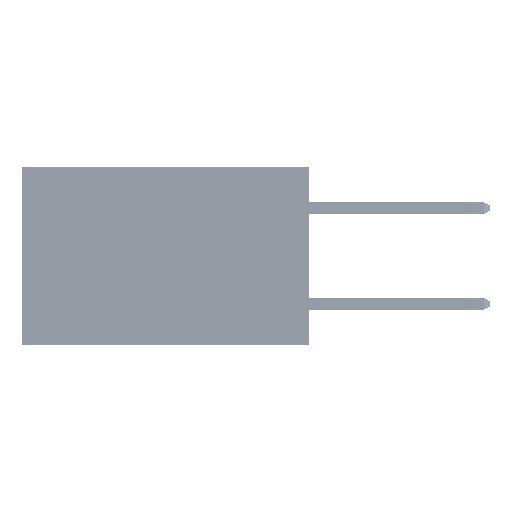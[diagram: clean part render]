
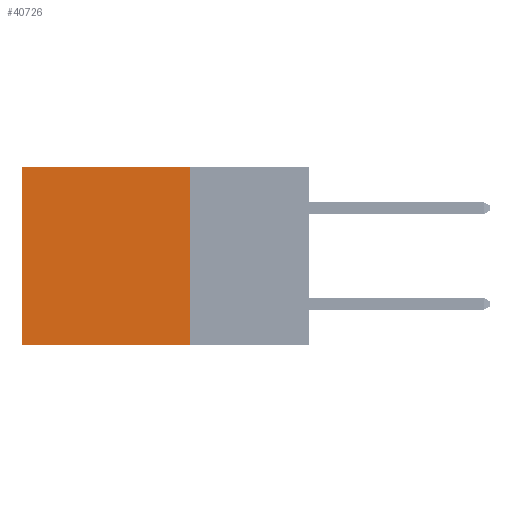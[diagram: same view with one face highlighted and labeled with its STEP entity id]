
A CAD part, left-side view. The second image highlights one B-rep face of the part: STEP entity #40726.
In plain terms, the highlighted planar face has unit normal (-1, 0, 0).
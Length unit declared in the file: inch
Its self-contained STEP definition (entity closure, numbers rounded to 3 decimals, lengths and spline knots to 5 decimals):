
#345 = ORIENTED_EDGE ( 'NONE', *, *, #44651, .F. ) ;
#456 = LINE ( 'NONE', #30104, #5459 ) ;
#1568 = CARTESIAN_POINT ( 'NONE',  ( 0.2875, 0.25, 0. ) ) ;
#2013 = LINE ( 'NONE', #16965, #23790 ) ;
#3012 = EDGE_LOOP ( 'NONE', ( #31496, #41289, #345, #5536 ) ) ;
#5459 = VECTOR ( 'NONE', #45035, 39.37008 ) ;
#5536 = ORIENTED_EDGE ( 'NONE', *, *, #22807, .T. ) ;
#8009 = VERTEX_POINT ( 'NONE', #40528 ) ;
#8767 = CARTESIAN_POINT ( 'NONE',  ( 0.2875, 0.25, -0.37 ) ) ;
#8848 = DIRECTION ( 'NONE',  ( 0., 0., -1. ) ) ;
#9375 = EDGE_CURVE ( 'NONE', #11975, #38595, #456, .T. ) ;
#11975 = VERTEX_POINT ( 'NONE', #8767 ) ;
#13280 = DIRECTION ( 'NONE',  ( 0., 0., -1. ) ) ;
#14042 = LINE ( 'NONE', #26265, #38725 ) ;
#16034 = DIRECTION ( 'NONE',  ( 0., 1., 0. ) ) ;
#16965 = CARTESIAN_POINT ( 'NONE',  ( 0.2875, 0.6, 0. ) ) ;
#17728 = DIRECTION ( 'NONE',  ( 0., 0., -1. ) ) ;
#22190 = CARTESIAN_POINT ( 'NONE',  ( 0.2875, 0.6, -0.37 ) ) ;
#22807 = EDGE_CURVE ( 'NONE', #28123, #8009, #42220, .T. ) ;
#23790 = VECTOR ( 'NONE', #13280, 39.37008 ) ;
#24289 = DIRECTION ( 'NONE',  ( 1., 0., 0. ) ) ;
#25136 = VECTOR ( 'NONE', #16034, 39.37008 ) ;
#26065 = EDGE_CURVE ( 'NONE', #8009, #38595, #2013, .T. ) ;
#26265 = CARTESIAN_POINT ( 'NONE',  ( 0.2875, 0.25, 0. ) ) ;
#27227 = CARTESIAN_POINT ( 'NONE',  ( 0.2875, 0.25, 0. ) ) ;
#28123 = VERTEX_POINT ( 'NONE', #35451 ) ;
#30104 = CARTESIAN_POINT ( 'NONE',  ( 0.2875, 0.25, -0.37 ) ) ;
#31496 = ORIENTED_EDGE ( 'NONE', *, *, #26065, .T. ) ;
#31552 = AXIS2_PLACEMENT_3D ( 'NONE', #27227, #24289, #8848 ) ;
#35451 = CARTESIAN_POINT ( 'NONE',  ( 0.2875, 0.25, 0. ) ) ;
#38474 = FACE_OUTER_BOUND ( 'NONE', #3012, .T. ) ;
#38595 = VERTEX_POINT ( 'NONE', #22190 ) ;
#38725 = VECTOR ( 'NONE', #17728, 39.37008 ) ;
#40528 = CARTESIAN_POINT ( 'NONE',  ( 0.2875, 0.6, 0. ) ) ;
#40726 = ADVANCED_FACE ( 'NONE', ( #38474 ), #42393, .F. ) ;
#41289 = ORIENTED_EDGE ( 'NONE', *, *, #9375, .F. ) ;
#42220 = LINE ( 'NONE', #1568, #25136 ) ;
#42393 = PLANE ( 'NONE',  #31552 ) ;
#44651 = EDGE_CURVE ( 'NONE', #28123, #11975, #14042, .T. ) ;
#45035 = DIRECTION ( 'NONE',  ( 0., 1., 0. ) ) ;
